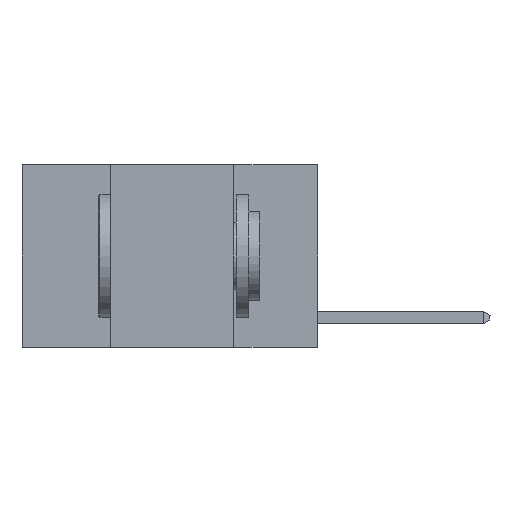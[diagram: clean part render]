
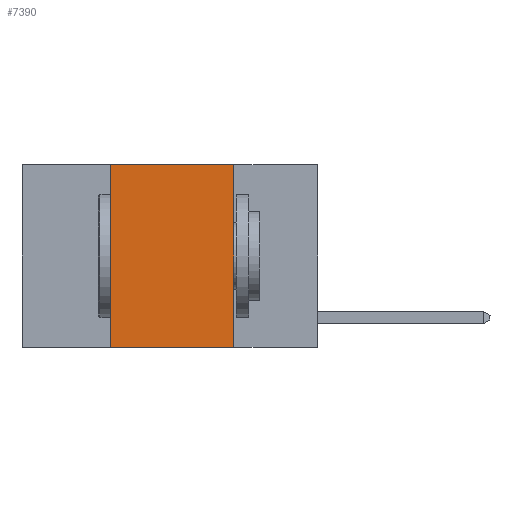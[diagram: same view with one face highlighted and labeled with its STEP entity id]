
A CAD part, left-side view. The second image highlights one B-rep face of the part: STEP entity #7390.
In plain terms, the highlighted planar face has unit normal (-1, 0, 0).
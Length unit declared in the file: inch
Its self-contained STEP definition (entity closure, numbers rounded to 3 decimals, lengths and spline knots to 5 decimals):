
#391 = LINE ( 'NONE', #1899, #8788 ) ;
#1162 = EDGE_LOOP ( 'NONE', ( #15898, #2866, #8836, #24008 ) ) ;
#1899 = CARTESIAN_POINT ( 'NONE',  ( 0., 0.6, -0.37 ) ) ;
#2866 = ORIENTED_EDGE ( 'NONE', *, *, #14160, .F. ) ;
#3371 = DIRECTION ( 'NONE',  ( 1., 0., 0. ) ) ;
#4391 = CARTESIAN_POINT ( 'NONE',  ( 0., 0.6, 0. ) ) ;
#4883 = VECTOR ( 'NONE', #20115, 39.37008 ) ;
#5285 = EDGE_CURVE ( 'NONE', #11911, #22916, #17945, .T. ) ;
#5882 = EDGE_CURVE ( 'NONE', #17048, #22916, #391, .T. ) ;
#5998 = CARTESIAN_POINT ( 'NONE',  ( 0., 0.17, 0. ) ) ;
#7390 = ADVANCED_FACE ( 'NONE', ( #11932 ), #10026, .F. ) ;
#7638 = CARTESIAN_POINT ( 'NONE',  ( 0., 0.17, 0. ) ) ;
#8321 = DIRECTION ( 'NONE',  ( 0., -1., 0. ) ) ;
#8788 = VECTOR ( 'NONE', #23059, 39.37008 ) ;
#8836 = ORIENTED_EDGE ( 'NONE', *, *, #10101, .F. ) ;
#8851 = LINE ( 'NONE', #4391, #12007 ) ;
#10026 = PLANE ( 'NONE',  #12339 ) ;
#10101 = EDGE_CURVE ( 'NONE', #17048, #18560, #14470, .T. ) ;
#11663 = CARTESIAN_POINT ( 'NONE',  ( 0., 0.6, 0. ) ) ;
#11790 = CARTESIAN_POINT ( 'NONE',  ( 0., 0.42, -0.37 ) ) ;
#11911 = VERTEX_POINT ( 'NONE', #5998 ) ;
#11932 = FACE_OUTER_BOUND ( 'NONE', #1162, .T. ) ;
#12007 = VECTOR ( 'NONE', #8321, 39.37008 ) ;
#12339 = AXIS2_PLACEMENT_3D ( 'NONE', #11663, #3371, #13818 ) ;
#13818 = DIRECTION ( 'NONE',  ( 0., 0., -1. ) ) ;
#14160 = EDGE_CURVE ( 'NONE', #18560, #11911, #8851, .T. ) ;
#14470 = LINE ( 'NONE', #24799, #20672 ) ;
#15898 = ORIENTED_EDGE ( 'NONE', *, *, #5285, .F. ) ;
#16760 = CARTESIAN_POINT ( 'NONE',  ( 0., 0.17, -0.37 ) ) ;
#17048 = VERTEX_POINT ( 'NONE', #11790 ) ;
#17945 = LINE ( 'NONE', #7638, #4883 ) ;
#18560 = VERTEX_POINT ( 'NONE', #26709 ) ;
#18810 = DIRECTION ( 'NONE',  ( 0., 0., 1. ) ) ;
#20115 = DIRECTION ( 'NONE',  ( 0., 0., -1. ) ) ;
#20672 = VECTOR ( 'NONE', #18810, 39.37008 ) ;
#22916 = VERTEX_POINT ( 'NONE', #16760 ) ;
#23059 = DIRECTION ( 'NONE',  ( 0., -1., 0. ) ) ;
#24008 = ORIENTED_EDGE ( 'NONE', *, *, #5882, .T. ) ;
#24799 = CARTESIAN_POINT ( 'NONE',  ( 0., 0.42, 0. ) ) ;
#26709 = CARTESIAN_POINT ( 'NONE',  ( 0., 0.42, 0. ) ) ;
